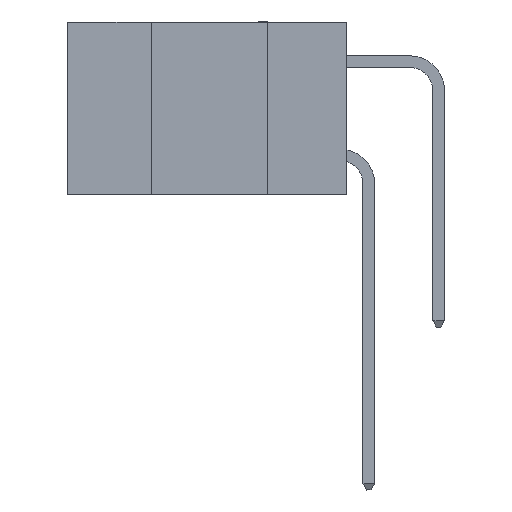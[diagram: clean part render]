
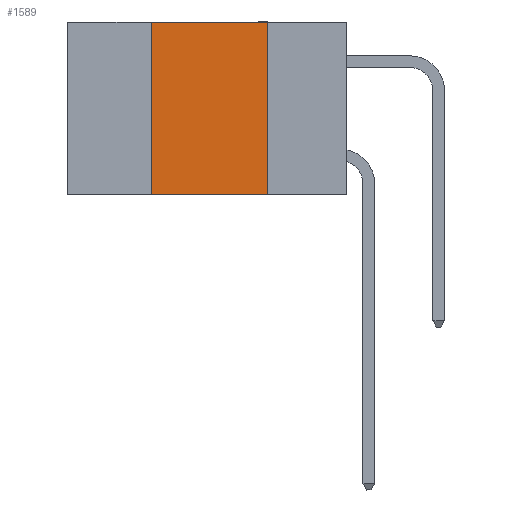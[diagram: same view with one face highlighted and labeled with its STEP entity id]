
A CAD part, left-side view. The second image highlights one B-rep face of the part: STEP entity #1589.
In plain terms, the highlighted planar face has unit normal (-1, 0, 0).
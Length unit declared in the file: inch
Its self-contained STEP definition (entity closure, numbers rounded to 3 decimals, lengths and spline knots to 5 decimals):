
#774 = VERTEX_POINT ( 'NONE', #11843 ) ;
#1589 = ADVANCED_FACE ( 'NONE', ( #19981 ), #28018, .F. ) ;
#1739 = LINE ( 'NONE', #2258, #34205 ) ;
#2258 = CARTESIAN_POINT ( 'NONE',  ( 0., 0.17, 0. ) ) ;
#2388 = EDGE_CURVE ( 'NONE', #28763, #10778, #29166, .T. ) ;
#3341 = VECTOR ( 'NONE', #18867, 39.37008 ) ;
#4289 = CARTESIAN_POINT ( 'NONE',  ( 0., 0.6, -0.37 ) ) ;
#4545 = ORIENTED_EDGE ( 'NONE', *, *, #28077, .F. ) ;
#6490 = AXIS2_PLACEMENT_3D ( 'NONE', #17189, #14728, #24898 ) ;
#8025 = CARTESIAN_POINT ( 'NONE',  ( 0., 0.17, 0. ) ) ;
#8419 = VECTOR ( 'NONE', #15090, 39.37008 ) ;
#9744 = CARTESIAN_POINT ( 'NONE',  ( 0., 0.17, -0.37 ) ) ;
#10778 = VERTEX_POINT ( 'NONE', #8025 ) ;
#11369 = ORIENTED_EDGE ( 'NONE', *, *, #25993, .T. ) ;
#11843 = CARTESIAN_POINT ( 'NONE',  ( 0., 0.42, -0.37 ) ) ;
#12928 = DIRECTION ( 'NONE',  ( 0., 0., -1. ) ) ;
#14728 = DIRECTION ( 'NONE',  ( 1., 0., 0. ) ) ;
#14950 = DIRECTION ( 'NONE',  ( 0., -1., 0. ) ) ;
#15090 = DIRECTION ( 'NONE',  ( 0., 0., 1. ) ) ;
#17189 = CARTESIAN_POINT ( 'NONE',  ( 0., 0.6, 0. ) ) ;
#18867 = DIRECTION ( 'NONE',  ( 0., -1., 0. ) ) ;
#18940 = ORIENTED_EDGE ( 'NONE', *, *, #2388, .F. ) ;
#19981 = FACE_OUTER_BOUND ( 'NONE', #26427, .T. ) ;
#20857 = LINE ( 'NONE', #31494, #8419 ) ;
#21497 = CARTESIAN_POINT ( 'NONE',  ( 0., 0.6, 0. ) ) ;
#21881 = VERTEX_POINT ( 'NONE', #9744 ) ;
#24898 = DIRECTION ( 'NONE',  ( 0., 0., -1. ) ) ;
#25993 = EDGE_CURVE ( 'NONE', #774, #21881, #28244, .T. ) ;
#26427 = EDGE_LOOP ( 'NONE', ( #4545, #18940, #34124, #11369 ) ) ;
#27076 = CARTESIAN_POINT ( 'NONE',  ( 0., 0.42, 0. ) ) ;
#28018 = PLANE ( 'NONE',  #6490 ) ;
#28077 = EDGE_CURVE ( 'NONE', #10778, #21881, #1739, .T. ) ;
#28244 = LINE ( 'NONE', #4289, #29506 ) ;
#28763 = VERTEX_POINT ( 'NONE', #27076 ) ;
#29166 = LINE ( 'NONE', #21497, #3341 ) ;
#29506 = VECTOR ( 'NONE', #14950, 39.37008 ) ;
#30998 = EDGE_CURVE ( 'NONE', #774, #28763, #20857, .T. ) ;
#31494 = CARTESIAN_POINT ( 'NONE',  ( 0., 0.42, 0. ) ) ;
#34124 = ORIENTED_EDGE ( 'NONE', *, *, #30998, .F. ) ;
#34205 = VECTOR ( 'NONE', #12928, 39.37008 ) ;
